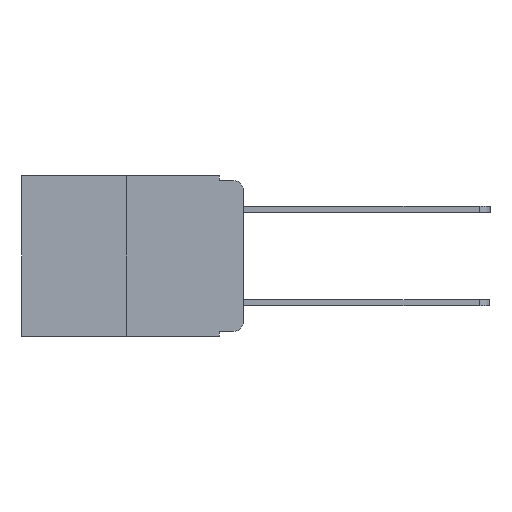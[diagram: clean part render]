
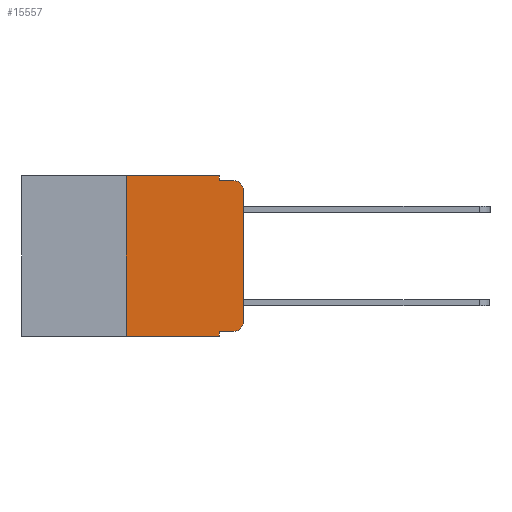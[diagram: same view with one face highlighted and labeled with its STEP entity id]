
A CAD part, left-side view. The second image highlights one B-rep face of the part: STEP entity #15557.
In plain terms, the highlighted planar face has unit normal (-1, 0, 0).
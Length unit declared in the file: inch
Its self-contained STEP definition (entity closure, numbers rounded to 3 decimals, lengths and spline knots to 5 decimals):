
#45 = EDGE_CURVE ( 'NONE', #7679, #21347, #367, .T. ) ;
#203 = LINE ( 'NONE', #2662, #5713 ) ;
#367 = LINE ( 'NONE', #15242, #10030 ) ;
#618 = VERTEX_POINT ( 'NONE', #22258 ) ;
#946 = ORIENTED_EDGE ( 'NONE', *, *, #5599, .T. ) ;
#1446 = EDGE_CURVE ( 'NONE', #21347, #13762, #24995, .T. ) ;
#1814 = VERTEX_POINT ( 'NONE', #25746 ) ;
#2258 = ORIENTED_EDGE ( 'NONE', *, *, #1446, .F. ) ;
#2431 = CIRCLE ( 'NONE', #22187, 0.02 ) ;
#2643 = VERTEX_POINT ( 'NONE', #14438 ) ;
#2662 = CARTESIAN_POINT ( 'NONE',  ( 0., 0.051, 0. ) ) ;
#2914 = ORIENTED_EDGE ( 'NONE', *, *, #45, .F. ) ;
#3468 = CARTESIAN_POINT ( 'NONE',  ( 0., 0.051, -0.333 ) ) ;
#3612 = CARTESIAN_POINT ( 'NONE',  ( 0., 0.02, -0.03 ) ) ;
#3865 = EDGE_LOOP ( 'NONE', ( #16133, #946, #2258, #2914, #4079, #13274, #16320, #6997, #24597, #7028 ) ) ;
#4079 = ORIENTED_EDGE ( 'NONE', *, *, #17504, .F. ) ;
#4876 = DIRECTION ( 'NONE',  ( 0., -1., 0. ) ) ;
#5081 = CARTESIAN_POINT ( 'NONE',  ( 0., 0.051, -0.01 ) ) ;
#5402 = AXIS2_PLACEMENT_3D ( 'NONE', #9112, #22855, #11102 ) ;
#5599 = EDGE_CURVE ( 'NONE', #1814, #13762, #7313, .T. ) ;
#5675 = DIRECTION ( 'NONE',  ( 0., 0., -1. ) ) ;
#5713 = VECTOR ( 'NONE', #14744, 39.37008 ) ;
#5949 = LINE ( 'NONE', #22748, #25702 ) ;
#6067 = CARTESIAN_POINT ( 'NONE',  ( 0., 0.051, 0. ) ) ;
#6114 = EDGE_CURVE ( 'NONE', #19509, #19694, #2431, .T. ) ;
#6739 = LINE ( 'NONE', #9377, #11490 ) ;
#6958 = EDGE_CURVE ( 'NONE', #19694, #1814, #9501, .T. ) ;
#6997 = ORIENTED_EDGE ( 'NONE', *, *, #12849, .F. ) ;
#7028 = ORIENTED_EDGE ( 'NONE', *, *, #6114, .T. ) ;
#7192 = FACE_OUTER_BOUND ( 'NONE', #3865, .T. ) ;
#7313 = CIRCLE ( 'NONE', #25740, 0.02 ) ;
#7679 = VERTEX_POINT ( 'NONE', #6067 ) ;
#8848 = DIRECTION ( 'NONE',  ( 0., -1., 0. ) ) ;
#8977 = CARTESIAN_POINT ( 'NONE',  ( 0., 0.051, -0.01 ) ) ;
#9112 = CARTESIAN_POINT ( 'NONE',  ( 0., 0.473, 0. ) ) ;
#9377 = CARTESIAN_POINT ( 'NONE',  ( 0., 0.473, 0. ) ) ;
#9501 = LINE ( 'NONE', #11909, #19373 ) ;
#9605 = CARTESIAN_POINT ( 'NONE',  ( 0., 0.02, -0.313 ) ) ;
#10030 = VECTOR ( 'NONE', #21000, 39.37008 ) ;
#10412 = VERTEX_POINT ( 'NONE', #3468 ) ;
#10965 = DIRECTION ( 'NONE',  ( 0., 0., 1. ) ) ;
#11019 = PLANE ( 'NONE',  #5402 ) ;
#11102 = DIRECTION ( 'NONE',  ( 0., 0., -1. ) ) ;
#11123 = CARTESIAN_POINT ( 'NONE',  ( 0., 0.02, -0.01 ) ) ;
#11490 = VECTOR ( 'NONE', #21161, 39.37008 ) ;
#11533 = EDGE_CURVE ( 'NONE', #10412, #19509, #22142, .T. ) ;
#11593 = DIRECTION ( 'NONE',  ( 0., 0., -1. ) ) ;
#11909 = CARTESIAN_POINT ( 'NONE',  ( 0., 0., 0. ) ) ;
#12127 = CARTESIAN_POINT ( 'NONE',  ( 0., 0.25, -0.343 ) ) ;
#12849 = EDGE_CURVE ( 'NONE', #10412, #2643, #203, .T. ) ;
#13274 = ORIENTED_EDGE ( 'NONE', *, *, #16797, .F. ) ;
#13762 = VERTEX_POINT ( 'NONE', #11123 ) ;
#14362 = EDGE_CURVE ( 'NONE', #25779, #2643, #5949, .T. ) ;
#14438 = CARTESIAN_POINT ( 'NONE',  ( 0., 0.051, -0.343 ) ) ;
#14744 = DIRECTION ( 'NONE',  ( 0., 0., -1. ) ) ;
#15242 = CARTESIAN_POINT ( 'NONE',  ( 0., 0.051, 0. ) ) ;
#15557 = ADVANCED_FACE ( 'NONE', ( #7192 ), #11019, .F. ) ;
#16133 = ORIENTED_EDGE ( 'NONE', *, *, #6958, .T. ) ;
#16320 = ORIENTED_EDGE ( 'NONE', *, *, #14362, .T. ) ;
#16797 = EDGE_CURVE ( 'NONE', #25779, #618, #23483, .T. ) ;
#16942 = VECTOR ( 'NONE', #8848, 39.37008 ) ;
#17504 = EDGE_CURVE ( 'NONE', #618, #7679, #6739, .T. ) ;
#17623 = DIRECTION ( 'NONE',  ( -1., 0., 0. ) ) ;
#18279 = VECTOR ( 'NONE', #10965, 39.37008 ) ;
#19206 = CARTESIAN_POINT ( 'NONE',  ( 0., 0.02, -0.333 ) ) ;
#19373 = VECTOR ( 'NONE', #23646, 39.37008 ) ;
#19509 = VERTEX_POINT ( 'NONE', #19206 ) ;
#19694 = VERTEX_POINT ( 'NONE', #21751 ) ;
#19823 = VECTOR ( 'NONE', #20789, 39.37008 ) ;
#20789 = DIRECTION ( 'NONE',  ( 0., -1., 0. ) ) ;
#21000 = DIRECTION ( 'NONE',  ( 0., 0., -1. ) ) ;
#21161 = DIRECTION ( 'NONE',  ( 0., -1., 0. ) ) ;
#21347 = VERTEX_POINT ( 'NONE', #5081 ) ;
#21751 = CARTESIAN_POINT ( 'NONE',  ( 0., 0., -0.313 ) ) ;
#22142 = LINE ( 'NONE', #22692, #16942 ) ;
#22187 = AXIS2_PLACEMENT_3D ( 'NONE', #9605, #23322, #11593 ) ;
#22258 = CARTESIAN_POINT ( 'NONE',  ( 0., 0.25, 0. ) ) ;
#22692 = CARTESIAN_POINT ( 'NONE',  ( 0., 0.051, -0.333 ) ) ;
#22693 = CARTESIAN_POINT ( 'NONE',  ( 0., 0.25, 0. ) ) ;
#22748 = CARTESIAN_POINT ( 'NONE',  ( 0., 0.473, -0.343 ) ) ;
#22855 = DIRECTION ( 'NONE',  ( 1., 0., 0. ) ) ;
#23322 = DIRECTION ( 'NONE',  ( -1., 0., 0. ) ) ;
#23483 = LINE ( 'NONE', #22693, #18279 ) ;
#23646 = DIRECTION ( 'NONE',  ( 0., 0., 1. ) ) ;
#24597 = ORIENTED_EDGE ( 'NONE', *, *, #11533, .T. ) ;
#24995 = LINE ( 'NONE', #8977, #19823 ) ;
#25702 = VECTOR ( 'NONE', #4876, 39.37008 ) ;
#25740 = AXIS2_PLACEMENT_3D ( 'NONE', #3612, #17623, #5675 ) ;
#25746 = CARTESIAN_POINT ( 'NONE',  ( 0., 0., -0.03 ) ) ;
#25779 = VERTEX_POINT ( 'NONE', #12127 ) ;
